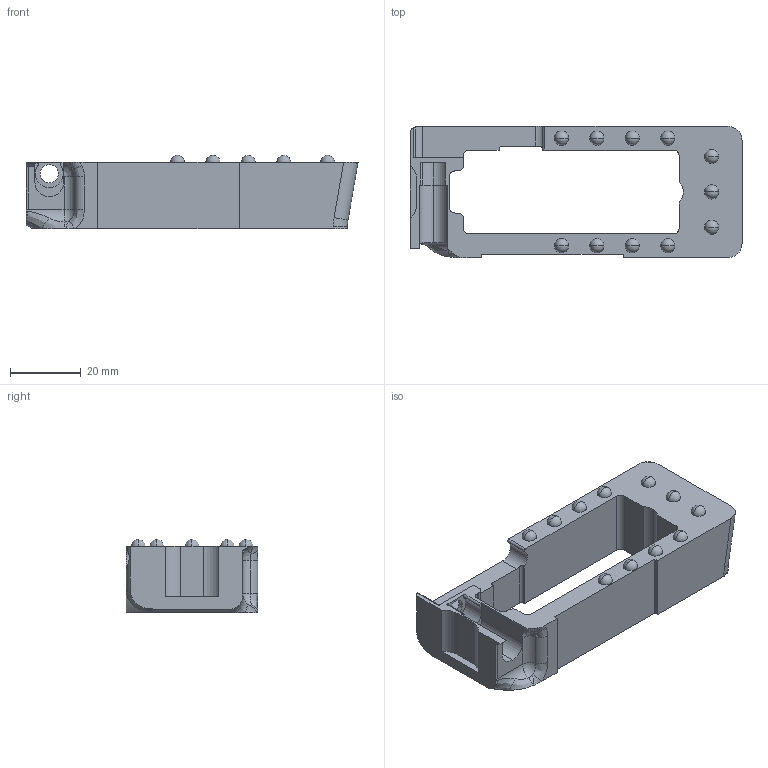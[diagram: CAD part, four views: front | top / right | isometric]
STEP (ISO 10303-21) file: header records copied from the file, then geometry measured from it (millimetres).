
FILE_DESCRIPTION (( 'STEP AP214' ), '1' );
FILE_NAME ('Magwell_2_1.step', '2019-12-18T03:08:13', ( '' ), ( '' ), 'SwSTEP 2.0', 'SolidWorks 2019', '' );
FILE_SCHEMA (( 'AUTOMOTIVE_DESIGN' ));
Length unit declared in the file: millimetre
Products named in the file (1): Magwell_2_1
Bounding box: 93.81 x 37.13 x 20.71 mm (x, y, z)
Volume: 30558 mm3; surface area: 11910.4 mm2
Topology: 1 solids, 1 shells, 122 faces, 366 edges, 234 vertices
Faces by surface type: cylinder 42, plane 34, sphere 24, bspline 15, torus 7
Entity records: 4647 total; most frequent: CARTESIAN_POINT 1620, ORIENTED_EDGE 642, DIRECTION 618, EDGE_CURVE 321, AXIS2_PLACEMENT_3D 242, VERTEX_POINT 212, EDGE_LOOP 137, VECTOR 134
